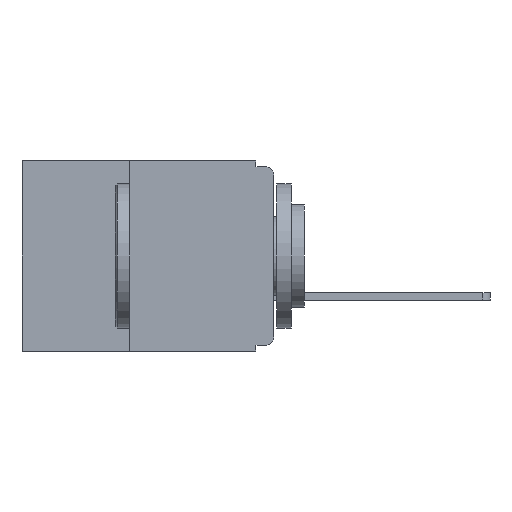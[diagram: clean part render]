
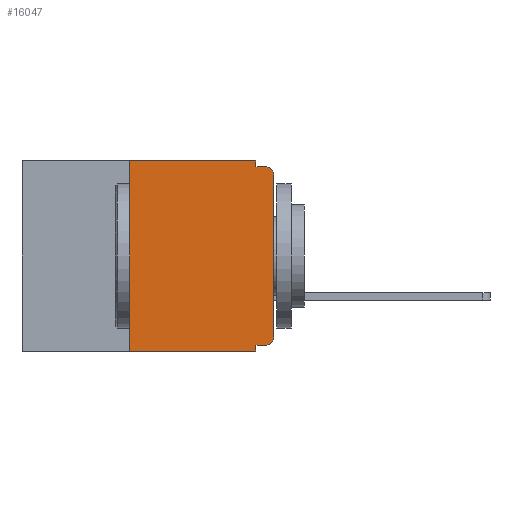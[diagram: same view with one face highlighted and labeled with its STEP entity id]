
A CAD part, left-side view. The second image highlights one B-rep face of the part: STEP entity #16047.
In plain terms, the highlighted planar face has unit normal (-1, 0, 0).
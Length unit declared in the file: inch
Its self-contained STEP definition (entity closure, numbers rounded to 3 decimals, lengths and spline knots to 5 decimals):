
#224 = CARTESIAN_POINT ( 'NONE',  ( 0., 0.031, 0. ) ) ;
#953 = CARTESIAN_POINT ( 'NONE',  ( 0., 0.437, -0.33 ) ) ;
#1140 = EDGE_CURVE ( 'NONE', #16050, #20486, #10365, .T. ) ;
#1345 = CARTESIAN_POINT ( 'NONE',  ( 0., 0.031, -0.32 ) ) ;
#1380 = EDGE_CURVE ( 'NONE', #20486, #1603, #20474, .T. ) ;
#1603 = VERTEX_POINT ( 'NONE', #17857 ) ;
#1680 = VECTOR ( 'NONE', #8157, 39.37008 ) ;
#1812 = CARTESIAN_POINT ( 'NONE',  ( 0., 0.437, 0. ) ) ;
#2283 = VERTEX_POINT ( 'NONE', #18745 ) ;
#2813 = ORIENTED_EDGE ( 'NONE', *, *, #1140, .F. ) ;
#3213 = CARTESIAN_POINT ( 'NONE',  ( 0., 0.031, 0. ) ) ;
#3311 = VECTOR ( 'NONE', #22037, 39.37008 ) ;
#3396 = VERTEX_POINT ( 'NONE', #5350 ) ;
#3451 = VERTEX_POINT ( 'NONE', #1345 ) ;
#3818 = CARTESIAN_POINT ( 'NONE',  ( 0., 0.031, -0.33 ) ) ;
#4278 = ORIENTED_EDGE ( 'NONE', *, *, #25024, .F. ) ;
#4366 = VERTEX_POINT ( 'NONE', #3818 ) ;
#4421 = VECTOR ( 'NONE', #12770, 39.37008 ) ;
#5350 = CARTESIAN_POINT ( 'NONE',  ( 0., 0., -0.305 ) ) ;
#5575 = EDGE_CURVE ( 'NONE', #2283, #1603, #8680, .T. ) ;
#5883 = CARTESIAN_POINT ( 'NONE',  ( 0., 0.015, -0.305 ) ) ;
#6093 = PLANE ( 'NONE',  #22383 ) ;
#6188 = CARTESIAN_POINT ( 'NONE',  ( 0., 0., -0.01 ) ) ;
#7024 = CARTESIAN_POINT ( 'NONE',  ( 0., 0.015, -0.32 ) ) ;
#7173 = VERTEX_POINT ( 'NONE', #9877 ) ;
#7310 = EDGE_CURVE ( 'NONE', #3396, #2283, #8582, .T. ) ;
#7387 = VECTOR ( 'NONE', #9758, 39.37008 ) ;
#7894 = DIRECTION ( 'NONE',  ( 0., 0., -1. ) ) ;
#8109 = DIRECTION ( 'NONE',  ( 1., 0., 0. ) ) ;
#8157 = DIRECTION ( 'NONE',  ( 0., 0., 1. ) ) ;
#8582 = LINE ( 'NONE', #12246, #3311 ) ;
#8680 = CIRCLE ( 'NONE', #21535, 0.015 ) ;
#8783 = VECTOR ( 'NONE', #13011, 39.37008 ) ;
#8925 = ORIENTED_EDGE ( 'NONE', *, *, #11095, .T. ) ;
#9124 = ORIENTED_EDGE ( 'NONE', *, *, #19041, .F. ) ;
#9640 = DIRECTION ( 'NONE',  ( 0., -1., 0. ) ) ;
#9665 = DIRECTION ( 'NONE',  ( 0., 0., -1. ) ) ;
#9670 = DIRECTION ( 'NONE',  ( -1., 0., 0. ) ) ;
#9717 = CARTESIAN_POINT ( 'NONE',  ( 0., 0.015, -0.025 ) ) ;
#9758 = DIRECTION ( 'NONE',  ( 0., 0., -1. ) ) ;
#9877 = CARTESIAN_POINT ( 'NONE',  ( 0., 0.25, 0. ) ) ;
#10365 = LINE ( 'NONE', #3213, #20802 ) ;
#11095 = EDGE_CURVE ( 'NONE', #12260, #3396, #14878, .T. ) ;
#11173 = ORIENTED_EDGE ( 'NONE', *, *, #25337, .F. ) ;
#12246 = CARTESIAN_POINT ( 'NONE',  ( 0., 0., 0. ) ) ;
#12260 = VERTEX_POINT ( 'NONE', #7024 ) ;
#12599 = LINE ( 'NONE', #21500, #7387 ) ;
#12770 = DIRECTION ( 'NONE',  ( 0., -1., 0. ) ) ;
#13011 = DIRECTION ( 'NONE',  ( 0., 1., 0. ) ) ;
#13263 = AXIS2_PLACEMENT_3D ( 'NONE', #5883, #19631, #7894 ) ;
#13986 = LINE ( 'NONE', #18836, #8783 ) ;
#14878 = CIRCLE ( 'NONE', #13263, 0.015 ) ;
#15094 = VERTEX_POINT ( 'NONE', #18751 ) ;
#15270 = VECTOR ( 'NONE', #9640, 39.37008 ) ;
#15448 = ORIENTED_EDGE ( 'NONE', *, *, #5575, .T. ) ;
#15642 = VECTOR ( 'NONE', #21520, 39.37008 ) ;
#16047 = ADVANCED_FACE ( 'NONE', ( #21263 ), #6093, .F. ) ;
#16050 = VERTEX_POINT ( 'NONE', #224 ) ;
#16540 = ORIENTED_EDGE ( 'NONE', *, *, #20824, .T. ) ;
#16582 = ORIENTED_EDGE ( 'NONE', *, *, #1380, .F. ) ;
#17187 = EDGE_CURVE ( 'NONE', #3451, #4366, #12599, .T. ) ;
#17857 = CARTESIAN_POINT ( 'NONE',  ( 0., 0.015, -0.01 ) ) ;
#18733 = ORIENTED_EDGE ( 'NONE', *, *, #17187, .F. ) ;
#18745 = CARTESIAN_POINT ( 'NONE',  ( 0., 0., -0.025 ) ) ;
#18751 = CARTESIAN_POINT ( 'NONE',  ( 0., 0.25, -0.33 ) ) ;
#18836 = CARTESIAN_POINT ( 'NONE',  ( 0., 0., -0.32 ) ) ;
#19041 = EDGE_CURVE ( 'NONE', #7173, #16050, #20840, .T. ) ;
#19631 = DIRECTION ( 'NONE',  ( -1., 0., 0. ) ) ;
#19839 = CARTESIAN_POINT ( 'NONE',  ( 0., 0.437, 0. ) ) ;
#20474 = LINE ( 'NONE', #6188, #15270 ) ;
#20486 = VERTEX_POINT ( 'NONE', #21449 ) ;
#20717 = ORIENTED_EDGE ( 'NONE', *, *, #7310, .T. ) ;
#20802 = VECTOR ( 'NONE', #23672, 39.37008 ) ;
#20803 = EDGE_LOOP ( 'NONE', ( #20717, #15448, #16582, #2813, #9124, #4278, #16540, #18733, #11173, #8925 ) ) ;
#20824 = EDGE_CURVE ( 'NONE', #15094, #4366, #25311, .T. ) ;
#20840 = LINE ( 'NONE', #1812, #15642 ) ;
#21263 = FACE_OUTER_BOUND ( 'NONE', #20803, .T. ) ;
#21375 = LINE ( 'NONE', #21867, #1680 ) ;
#21449 = CARTESIAN_POINT ( 'NONE',  ( 0., 0.031, -0.01 ) ) ;
#21500 = CARTESIAN_POINT ( 'NONE',  ( 0., 0.031, -0.33 ) ) ;
#21520 = DIRECTION ( 'NONE',  ( 0., -1., 0. ) ) ;
#21535 = AXIS2_PLACEMENT_3D ( 'NONE', #9717, #9670, #9665 ) ;
#21812 = DIRECTION ( 'NONE',  ( 0., 0., -1. ) ) ;
#21867 = CARTESIAN_POINT ( 'NONE',  ( 0., 0.25, -0.33 ) ) ;
#22037 = DIRECTION ( 'NONE',  ( 0., 0., 1. ) ) ;
#22383 = AXIS2_PLACEMENT_3D ( 'NONE', #19839, #8109, #21812 ) ;
#23672 = DIRECTION ( 'NONE',  ( 0., 0., -1. ) ) ;
#25024 = EDGE_CURVE ( 'NONE', #15094, #7173, #21375, .T. ) ;
#25311 = LINE ( 'NONE', #953, #4421 ) ;
#25337 = EDGE_CURVE ( 'NONE', #12260, #3451, #13986, .T. ) ;
